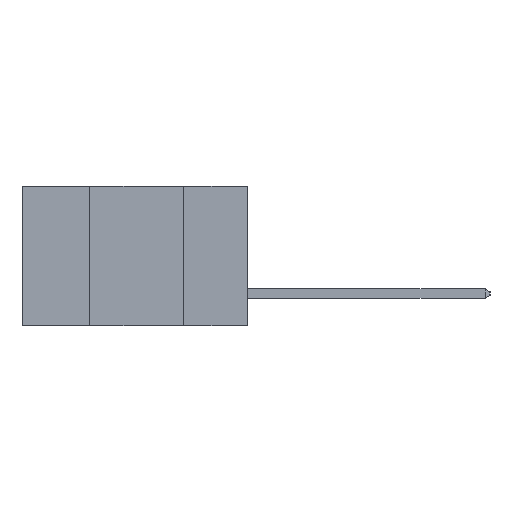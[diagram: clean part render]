
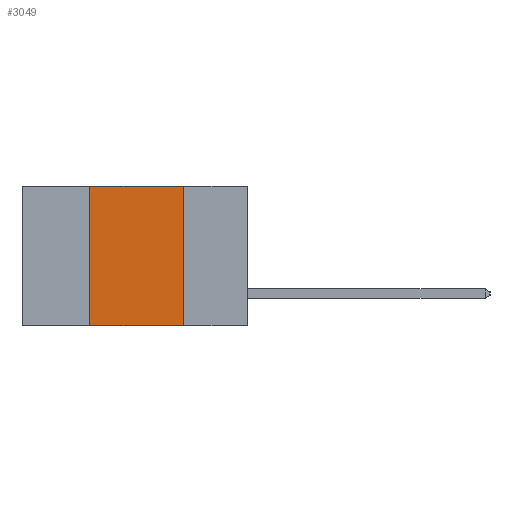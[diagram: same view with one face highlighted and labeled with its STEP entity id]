
A CAD part, left-side view. The second image highlights one B-rep face of the part: STEP entity #3049.
In plain terms, the highlighted planar face has unit normal (-1, 0, 0).
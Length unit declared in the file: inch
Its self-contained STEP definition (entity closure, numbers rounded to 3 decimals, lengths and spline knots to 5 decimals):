
#299 = CARTESIAN_POINT ( 'NONE',  ( 0., 0.17, 0. ) ) ;
#1231 = CARTESIAN_POINT ( 'NONE',  ( 0., 0.17, -0.37 ) ) ;
#2154 = VECTOR ( 'NONE', #15086, 39.37008 ) ;
#2454 = VERTEX_POINT ( 'NONE', #9479 ) ;
#3049 = ADVANCED_FACE ( 'NONE', ( #12909 ), #15635, .F. ) ;
#3505 = ORIENTED_EDGE ( 'NONE', *, *, #9921, .F. ) ;
#3582 = LINE ( 'NONE', #6681, #20719 ) ;
#4362 = LINE ( 'NONE', #13478, #12839 ) ;
#4892 = DIRECTION ( 'NONE',  ( 0., -1., 0. ) ) ;
#6681 = CARTESIAN_POINT ( 'NONE',  ( 0., 0.6, 0. ) ) ;
#6968 = ORIENTED_EDGE ( 'NONE', *, *, #15229, .F. ) ;
#8560 = DIRECTION ( 'NONE',  ( 0., 0., 1. ) ) ;
#8936 = EDGE_CURVE ( 'NONE', #2454, #10711, #11166, .T. ) ;
#9283 = VECTOR ( 'NONE', #8560, 39.37008 ) ;
#9415 = AXIS2_PLACEMENT_3D ( 'NONE', #15776, #15631, #15607 ) ;
#9479 = CARTESIAN_POINT ( 'NONE',  ( 0., 0.42, -0.37 ) ) ;
#9801 = VERTEX_POINT ( 'NONE', #299 ) ;
#9921 = EDGE_CURVE ( 'NONE', #2454, #17031, #13711, .T. ) ;
#10711 = VERTEX_POINT ( 'NONE', #1231 ) ;
#10982 = CARTESIAN_POINT ( 'NONE',  ( 0., 0.42, 0. ) ) ;
#11166 = LINE ( 'NONE', #15113, #2154 ) ;
#12839 = VECTOR ( 'NONE', #13195, 39.37008 ) ;
#12909 = FACE_OUTER_BOUND ( 'NONE', #16783, .T. ) ;
#13195 = DIRECTION ( 'NONE',  ( 0., 0., -1. ) ) ;
#13349 = CARTESIAN_POINT ( 'NONE',  ( 0., 0.42, -0.37 ) ) ;
#13478 = CARTESIAN_POINT ( 'NONE',  ( 0., 0.17, -0.37 ) ) ;
#13711 = LINE ( 'NONE', #13349, #9283 ) ;
#15086 = DIRECTION ( 'NONE',  ( 0., -1., 0. ) ) ;
#15113 = CARTESIAN_POINT ( 'NONE',  ( 0., 0.6, -0.37 ) ) ;
#15229 = EDGE_CURVE ( 'NONE', #17031, #9801, #3582, .T. ) ;
#15607 = DIRECTION ( 'NONE',  ( 0., 0., -1. ) ) ;
#15631 = DIRECTION ( 'NONE',  ( 1., 0., 0. ) ) ;
#15633 = EDGE_CURVE ( 'NONE', #9801, #10711, #4362, .T. ) ;
#15635 = PLANE ( 'NONE',  #9415 ) ;
#15776 = CARTESIAN_POINT ( 'NONE',  ( 0., 0.6, 0. ) ) ;
#15837 = ORIENTED_EDGE ( 'NONE', *, *, #15633, .F. ) ;
#16783 = EDGE_LOOP ( 'NONE', ( #15837, #6968, #3505, #20662 ) ) ;
#17031 = VERTEX_POINT ( 'NONE', #10982 ) ;
#20662 = ORIENTED_EDGE ( 'NONE', *, *, #8936, .T. ) ;
#20719 = VECTOR ( 'NONE', #4892, 39.37008 ) ;
